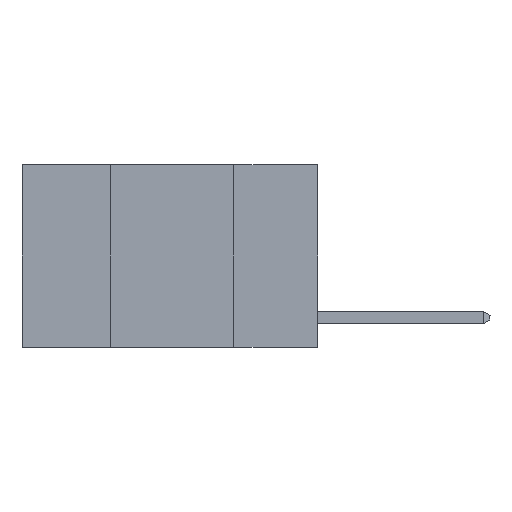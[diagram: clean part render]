
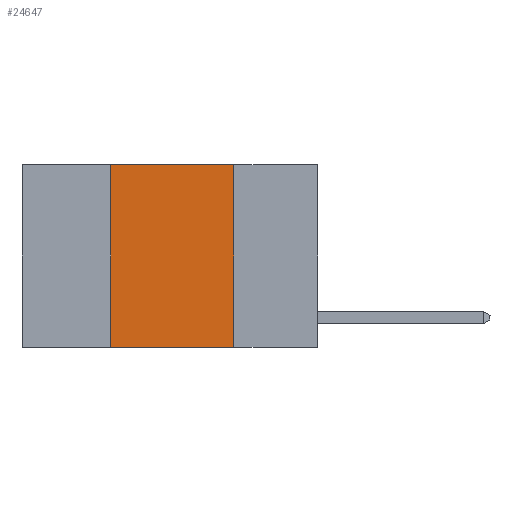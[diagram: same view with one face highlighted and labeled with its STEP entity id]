
A CAD part, left-side view. The second image highlights one B-rep face of the part: STEP entity #24647.
In plain terms, the highlighted planar face has unit normal (-1, 0, 0).
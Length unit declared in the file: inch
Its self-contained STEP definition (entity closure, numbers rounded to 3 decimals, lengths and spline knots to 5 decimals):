
#140 = DIRECTION ( 'NONE',  ( 0., -1., 0. ) ) ;
#295 = CARTESIAN_POINT ( 'NONE',  ( 0., 0.17, 0. ) ) ;
#1520 = CARTESIAN_POINT ( 'NONE',  ( 0., 0.42, 0. ) ) ;
#1952 = DIRECTION ( 'NONE',  ( 0., 0., -1. ) ) ;
#2648 = ORIENTED_EDGE ( 'NONE', *, *, #13853, .T. ) ;
#2888 = FACE_OUTER_BOUND ( 'NONE', #14427, .T. ) ;
#3423 = VERTEX_POINT ( 'NONE', #9032 ) ;
#3958 = VECTOR ( 'NONE', #21750, 39.37008 ) ;
#4110 = VECTOR ( 'NONE', #140, 39.37008 ) ;
#4844 = LINE ( 'NONE', #19212, #4110 ) ;
#5043 = CARTESIAN_POINT ( 'NONE',  ( 0., 0.17, 0. ) ) ;
#9032 = CARTESIAN_POINT ( 'NONE',  ( 0., 0.42, -0.37 ) ) ;
#9849 = CARTESIAN_POINT ( 'NONE',  ( 0., 0.6, 0. ) ) ;
#10819 = ORIENTED_EDGE ( 'NONE', *, *, #20264, .F. ) ;
#13040 = ORIENTED_EDGE ( 'NONE', *, *, #22137, .F. ) ;
#13808 = CARTESIAN_POINT ( 'NONE',  ( 0., 0.6, 0. ) ) ;
#13853 = EDGE_CURVE ( 'NONE', #3423, #30622, #4844, .T. ) ;
#14427 = EDGE_LOOP ( 'NONE', ( #10819, #13040, #20935, #2648 ) ) ;
#15230 = LINE ( 'NONE', #5043, #22330 ) ;
#15467 = EDGE_CURVE ( 'NONE', #3423, #27465, #20441, .T. ) ;
#16225 = DIRECTION ( 'NONE',  ( 1., 0., 0. ) ) ;
#18649 = AXIS2_PLACEMENT_3D ( 'NONE', #13808, #16225, #1952 ) ;
#19212 = CARTESIAN_POINT ( 'NONE',  ( 0., 0.6, -0.37 ) ) ;
#19671 = VECTOR ( 'NONE', #25377, 39.37008 ) ;
#19906 = CARTESIAN_POINT ( 'NONE',  ( 0., 0.17, -0.37 ) ) ;
#20264 = EDGE_CURVE ( 'NONE', #24208, #30622, #15230, .T. ) ;
#20441 = LINE ( 'NONE', #1520, #19671 ) ;
#20566 = CARTESIAN_POINT ( 'NONE',  ( 0., 0.42, 0. ) ) ;
#20935 = ORIENTED_EDGE ( 'NONE', *, *, #15467, .F. ) ;
#21750 = DIRECTION ( 'NONE',  ( 0., -1., 0. ) ) ;
#22137 = EDGE_CURVE ( 'NONE', #27465, #24208, #22969, .T. ) ;
#22330 = VECTOR ( 'NONE', #24124, 39.37008 ) ;
#22969 = LINE ( 'NONE', #9849, #3958 ) ;
#23285 = PLANE ( 'NONE',  #18649 ) ;
#24124 = DIRECTION ( 'NONE',  ( 0., 0., -1. ) ) ;
#24208 = VERTEX_POINT ( 'NONE', #295 ) ;
#24647 = ADVANCED_FACE ( 'NONE', ( #2888 ), #23285, .F. ) ;
#25377 = DIRECTION ( 'NONE',  ( 0., 0., 1. ) ) ;
#27465 = VERTEX_POINT ( 'NONE', #20566 ) ;
#30622 = VERTEX_POINT ( 'NONE', #19906 ) ;
